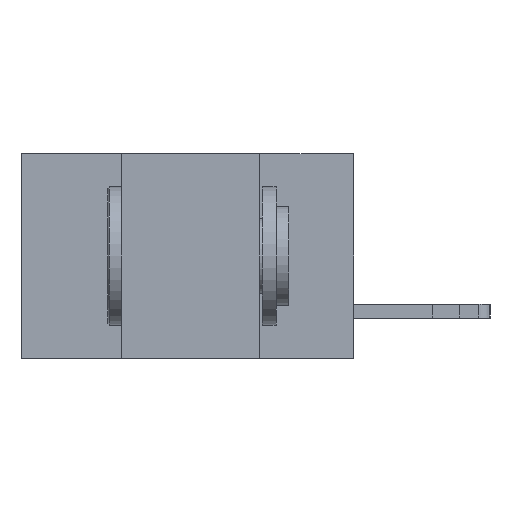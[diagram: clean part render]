
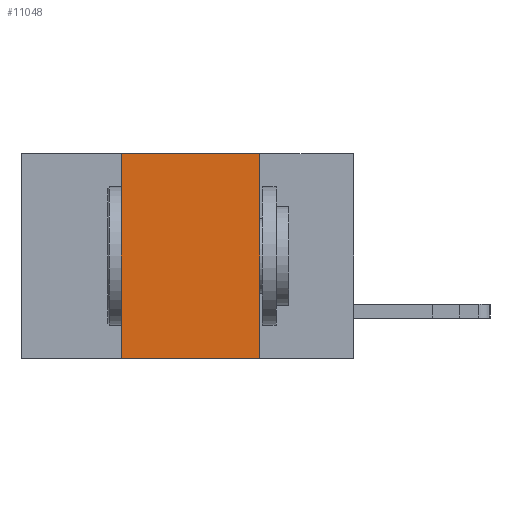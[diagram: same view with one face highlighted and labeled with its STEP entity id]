
A CAD part, left-side view. The second image highlights one B-rep face of the part: STEP entity #11048.
In plain terms, the highlighted planar face has unit normal (-1, 0, 0).
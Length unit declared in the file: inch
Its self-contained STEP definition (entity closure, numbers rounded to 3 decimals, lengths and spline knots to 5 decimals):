
#142 = FACE_OUTER_BOUND ( 'NONE', #13432, .T. ) ;
#301 = DIRECTION ( 'NONE',  ( 0., 0., 1. ) ) ;
#1666 = CARTESIAN_POINT ( 'NONE',  ( 0., 0.6, -0.37 ) ) ;
#3215 = LINE ( 'NONE', #12674, #5676 ) ;
#3977 = EDGE_CURVE ( 'NONE', #10033, #11001, #17318, .T. ) ;
#4264 = ORIENTED_EDGE ( 'NONE', *, *, #3977, .T. ) ;
#4273 = DIRECTION ( 'NONE',  ( 0., 0., -1. ) ) ;
#5558 = ORIENTED_EDGE ( 'NONE', *, *, #6532, .F. ) ;
#5676 = VECTOR ( 'NONE', #301, 39.37008 ) ;
#5745 = CARTESIAN_POINT ( 'NONE',  ( 0., 0.6, 0. ) ) ;
#5757 = EDGE_CURVE ( 'NONE', #10230, #16947, #10516, .T. ) ;
#6178 = ORIENTED_EDGE ( 'NONE', *, *, #5757, .F. ) ;
#6293 = DIRECTION ( 'NONE',  ( 0., -1., 0. ) ) ;
#6532 = EDGE_CURVE ( 'NONE', #10033, #10230, #3215, .T. ) ;
#6649 = ORIENTED_EDGE ( 'NONE', *, *, #7061, .F. ) ;
#7061 = EDGE_CURVE ( 'NONE', #16947, #11001, #13078, .T. ) ;
#7249 = DIRECTION ( 'NONE',  ( 0., -1., 0. ) ) ;
#9032 = AXIS2_PLACEMENT_3D ( 'NONE', #5745, #15359, #4273 ) ;
#9827 = DIRECTION ( 'NONE',  ( 0., 0., -1. ) ) ;
#10033 = VERTEX_POINT ( 'NONE', #14330 ) ;
#10230 = VERTEX_POINT ( 'NONE', #16437 ) ;
#10516 = LINE ( 'NONE', #13247, #10817 ) ;
#10817 = VECTOR ( 'NONE', #6293, 39.37008 ) ;
#11001 = VERTEX_POINT ( 'NONE', #14638 ) ;
#11048 = ADVANCED_FACE ( 'NONE', ( #142 ), #13979, .F. ) ;
#11245 = VECTOR ( 'NONE', #9827, 39.37008 ) ;
#11719 = CARTESIAN_POINT ( 'NONE',  ( 0., 0.17, 0. ) ) ;
#12674 = CARTESIAN_POINT ( 'NONE',  ( 0., 0.42, 0. ) ) ;
#13078 = LINE ( 'NONE', #11719, #11245 ) ;
#13247 = CARTESIAN_POINT ( 'NONE',  ( 0., 0.6, 0. ) ) ;
#13432 = EDGE_LOOP ( 'NONE', ( #6649, #6178, #5558, #4264 ) ) ;
#13979 = PLANE ( 'NONE',  #9032 ) ;
#14330 = CARTESIAN_POINT ( 'NONE',  ( 0., 0.42, -0.37 ) ) ;
#14638 = CARTESIAN_POINT ( 'NONE',  ( 0., 0.17, -0.37 ) ) ;
#15359 = DIRECTION ( 'NONE',  ( 1., 0., 0. ) ) ;
#16437 = CARTESIAN_POINT ( 'NONE',  ( 0., 0.42, 0. ) ) ;
#16947 = VERTEX_POINT ( 'NONE', #17792 ) ;
#17318 = LINE ( 'NONE', #1666, #17553 ) ;
#17553 = VECTOR ( 'NONE', #7249, 39.37008 ) ;
#17792 = CARTESIAN_POINT ( 'NONE',  ( 0., 0.17, 0. ) ) ;
